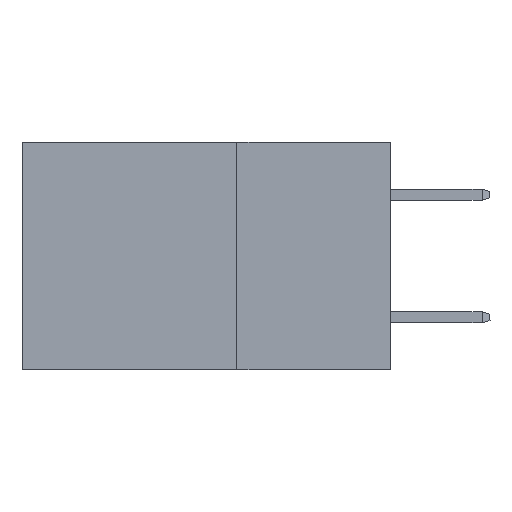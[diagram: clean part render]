
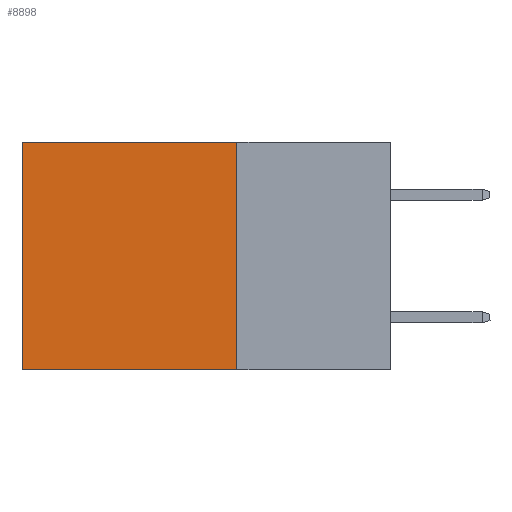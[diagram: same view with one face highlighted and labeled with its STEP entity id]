
A CAD part, left-side view. The second image highlights one B-rep face of the part: STEP entity #8898.
In plain terms, the highlighted planar face has unit normal (-1, 0, 0).
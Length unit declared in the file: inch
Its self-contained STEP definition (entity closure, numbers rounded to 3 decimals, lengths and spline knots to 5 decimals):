
#8 = EDGE_CURVE ( 'NONE', #10233, #12037, #17192, .T. ) ;
#111 = EDGE_LOOP ( 'NONE', ( #14666, #249, #749, #13636 ) ) ;
#249 = ORIENTED_EDGE ( 'NONE', *, *, #6926, .F. ) ;
#749 = ORIENTED_EDGE ( 'NONE', *, *, #1554, .F. ) ;
#1260 = CARTESIAN_POINT ( 'NONE',  ( 0.2875, 0.25, 0. ) ) ;
#1554 = EDGE_CURVE ( 'NONE', #10233, #2296, #8006, .T. ) ;
#1936 = CARTESIAN_POINT ( 'NONE',  ( 0.2875, 0.6, -0.37 ) ) ;
#2296 = VERTEX_POINT ( 'NONE', #15760 ) ;
#3126 = CARTESIAN_POINT ( 'NONE',  ( 0.2875, 0.25, 0. ) ) ;
#4685 = DIRECTION ( 'NONE',  ( 0., 0., -1. ) ) ;
#5815 = CARTESIAN_POINT ( 'NONE',  ( 0.2875, 0.6, 0. ) ) ;
#6708 = AXIS2_PLACEMENT_3D ( 'NONE', #3126, #13124, #4685 ) ;
#6926 = EDGE_CURVE ( 'NONE', #2296, #14983, #15634, .T. ) ;
#7279 = DIRECTION ( 'NONE',  ( 0., 0., -1. ) ) ;
#7551 = CARTESIAN_POINT ( 'NONE',  ( 0.2875, 0.6, 0. ) ) ;
#8006 = LINE ( 'NONE', #1260, #15378 ) ;
#8786 = CARTESIAN_POINT ( 'NONE',  ( 0.2875, 0.25, -0.37 ) ) ;
#8898 = ADVANCED_FACE ( 'NONE', ( #13370 ), #10341, .F. ) ;
#9021 = DIRECTION ( 'NONE',  ( 0., 1., 0. ) ) ;
#10233 = VERTEX_POINT ( 'NONE', #17218 ) ;
#10341 = PLANE ( 'NONE',  #6708 ) ;
#11500 = DIRECTION ( 'NONE',  ( 0., 0., -1. ) ) ;
#11901 = VECTOR ( 'NONE', #17098, 39.37008 ) ;
#12037 = VERTEX_POINT ( 'NONE', #7551 ) ;
#13124 = DIRECTION ( 'NONE',  ( 1., 0., 0. ) ) ;
#13370 = FACE_OUTER_BOUND ( 'NONE', #111, .T. ) ;
#13479 = VECTOR ( 'NONE', #9021, 39.37008 ) ;
#13636 = ORIENTED_EDGE ( 'NONE', *, *, #8, .T. ) ;
#14666 = ORIENTED_EDGE ( 'NONE', *, *, #15576, .T. ) ;
#14702 = LINE ( 'NONE', #5815, #17535 ) ;
#14983 = VERTEX_POINT ( 'NONE', #1936 ) ;
#15378 = VECTOR ( 'NONE', #11500, 39.37008 ) ;
#15576 = EDGE_CURVE ( 'NONE', #12037, #14983, #14702, .T. ) ;
#15634 = LINE ( 'NONE', #8786, #11901 ) ;
#15760 = CARTESIAN_POINT ( 'NONE',  ( 0.2875, 0.25, -0.37 ) ) ;
#16374 = CARTESIAN_POINT ( 'NONE',  ( 0.2875, 0.25, 0. ) ) ;
#17098 = DIRECTION ( 'NONE',  ( 0., 1., 0. ) ) ;
#17192 = LINE ( 'NONE', #16374, #13479 ) ;
#17218 = CARTESIAN_POINT ( 'NONE',  ( 0.2875, 0.25, 0. ) ) ;
#17535 = VECTOR ( 'NONE', #7279, 39.37008 ) ;
